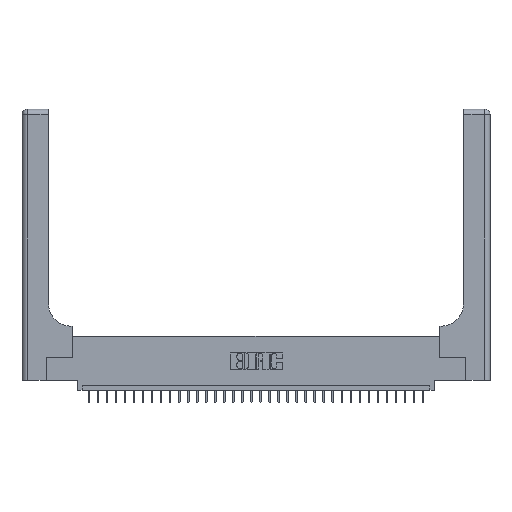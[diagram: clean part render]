
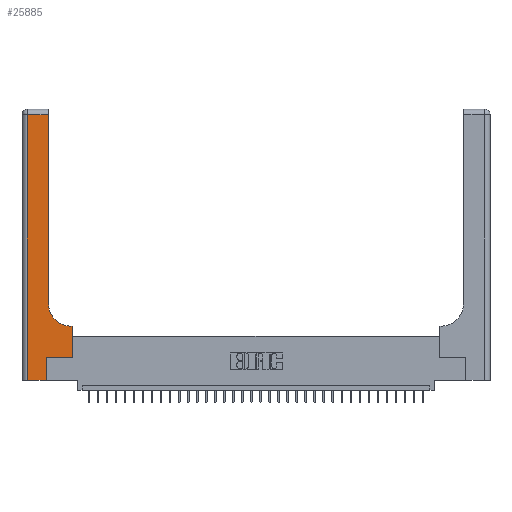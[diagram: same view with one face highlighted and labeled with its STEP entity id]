
A CAD part, top view. The second image highlights one B-rep face of the part: STEP entity #25885.
In plain terms, the highlighted planar face has unit normal (0, 0, 1).
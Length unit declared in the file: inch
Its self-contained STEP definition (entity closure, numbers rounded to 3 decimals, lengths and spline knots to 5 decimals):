
#152 = CARTESIAN_POINT ( 'NONE',  ( 0.2915, 0.6, 0.37 ) ) ;
#460 = EDGE_LOOP ( 'NONE', ( #8444, #33985, #28691, #29464, #1992, #9647, #3432, #23679, #12489 ) ) ;
#1067 = LINE ( 'NONE', #4034, #13639 ) ;
#1220 = EDGE_CURVE ( 'NONE', #16146, #11317, #33413, .T. ) ;
#1992 = ORIENTED_EDGE ( 'NONE', *, *, #14530, .T. ) ;
#2095 = CARTESIAN_POINT ( 'NONE',  ( 0.5585, 0.6, 0.37 ) ) ;
#3432 = ORIENTED_EDGE ( 'NONE', *, *, #22307, .T. ) ;
#3467 = DIRECTION ( 'NONE',  ( -1., 0., 0. ) ) ;
#3985 = EDGE_CURVE ( 'NONE', #18827, #16146, #16066, .T. ) ;
#3989 = VERTEX_POINT ( 'NONE', #16239 ) ;
#4034 = CARTESIAN_POINT ( 'NONE',  ( 0.2915, 3., 0.37 ) ) ;
#4475 = CARTESIAN_POINT ( 'NONE',  ( 0.5585, 0.25, 0.37 ) ) ;
#4802 = VERTEX_POINT ( 'NONE', #25611 ) ;
#5117 = CARTESIAN_POINT ( 'NONE',  ( 0.5415, 0.6, 0.37 ) ) ;
#5521 = VECTOR ( 'NONE', #21735, 39.37008 ) ;
#6195 = VECTOR ( 'NONE', #20926, 39.37008 ) ;
#6320 = LINE ( 'NONE', #27493, #5521 ) ;
#6955 = DIRECTION ( 'NONE',  ( -1., 0., 0. ) ) ;
#7333 = DIRECTION ( 'NONE',  ( 0., 0., -1. ) ) ;
#8444 = ORIENTED_EDGE ( 'NONE', *, *, #17525, .T. ) ;
#9647 = ORIENTED_EDGE ( 'NONE', *, *, #22580, .T. ) ;
#11091 = DIRECTION ( 'NONE',  ( 1., 0., 0. ) ) ;
#11154 = CARTESIAN_POINT ( 'NONE',  ( 0.06, 2.94, 0.37 ) ) ;
#11214 = EDGE_CURVE ( 'NONE', #3989, #29054, #6320, .T. ) ;
#11317 = VERTEX_POINT ( 'NONE', #25552 ) ;
#12489 = ORIENTED_EDGE ( 'NONE', *, *, #1220, .T. ) ;
#13508 = VERTEX_POINT ( 'NONE', #31583 ) ;
#13549 = EDGE_CURVE ( 'NONE', #13508, #22696, #31760, .T. ) ;
#13639 = VECTOR ( 'NONE', #27651, 39.37008 ) ;
#14232 = LINE ( 'NONE', #24223, #28880 ) ;
#14388 = CARTESIAN_POINT ( 'NONE',  ( 0.269, 0., 0.37 ) ) ;
#14448 = LINE ( 'NONE', #4475, #17110 ) ;
#14530 = EDGE_CURVE ( 'NONE', #22696, #4802, #32590, .T. ) ;
#14735 = CARTESIAN_POINT ( 'NONE',  ( 0.06, 3., 0.37 ) ) ;
#15183 = FACE_OUTER_BOUND ( 'NONE', #460, .T. ) ;
#15884 = EDGE_CURVE ( 'NONE', #29054, #13508, #17178, .T. ) ;
#16066 = LINE ( 'NONE', #152, #20074 ) ;
#16146 = VERTEX_POINT ( 'NONE', #5117 ) ;
#16239 = CARTESIAN_POINT ( 'NONE',  ( 0.2915, 2.94, 0.37 ) ) ;
#17110 = VECTOR ( 'NONE', #17749, 39.37008 ) ;
#17178 = LINE ( 'NONE', #14735, #30311 ) ;
#17525 = EDGE_CURVE ( 'NONE', #11317, #3989, #1067, .T. ) ;
#17749 = DIRECTION ( 'NONE',  ( 0., 1., 0. ) ) ;
#18466 = CARTESIAN_POINT ( 'NONE',  ( 0., 0., 0.37 ) ) ;
#18827 = VERTEX_POINT ( 'NONE', #2095 ) ;
#20074 = VECTOR ( 'NONE', #3467, 39.37008 ) ;
#20926 = DIRECTION ( 'NONE',  ( 1., 0., 0. ) ) ;
#21735 = DIRECTION ( 'NONE',  ( -1., 0., 0. ) ) ;
#21893 = VECTOR ( 'NONE', #22095, 39.37008 ) ;
#22095 = DIRECTION ( 'NONE',  ( 0., 1., 0. ) ) ;
#22205 = CARTESIAN_POINT ( 'NONE',  ( 0.5585, 0.25, 0.37 ) ) ;
#22307 = EDGE_CURVE ( 'NONE', #24770, #18827, #14448, .T. ) ;
#22580 = EDGE_CURVE ( 'NONE', #4802, #24770, #14232, .T. ) ;
#22696 = VERTEX_POINT ( 'NONE', #25415 ) ;
#22881 = PLANE ( 'NONE',  #33135 ) ;
#23679 = ORIENTED_EDGE ( 'NONE', *, *, #3985, .T. ) ;
#23955 = AXIS2_PLACEMENT_3D ( 'NONE', #31287, #7333, #28835 ) ;
#24223 = CARTESIAN_POINT ( 'NONE',  ( 0.269, 0.25, 0.37 ) ) ;
#24770 = VERTEX_POINT ( 'NONE', #22205 ) ;
#25415 = CARTESIAN_POINT ( 'NONE',  ( 0.269, 0., 0.37 ) ) ;
#25552 = CARTESIAN_POINT ( 'NONE',  ( 0.2915, 0.85, 0.37 ) ) ;
#25611 = CARTESIAN_POINT ( 'NONE',  ( 0.269, 0.25, 0.37 ) ) ;
#25885 = ADVANCED_FACE ( 'NONE', ( #15183 ), #22881, .F. ) ;
#27493 = CARTESIAN_POINT ( 'NONE',  ( 0., 2.94, 0.37 ) ) ;
#27651 = DIRECTION ( 'NONE',  ( 0., 1., 0. ) ) ;
#28691 = ORIENTED_EDGE ( 'NONE', *, *, #15884, .T. ) ;
#28835 = DIRECTION ( 'NONE',  ( 1., 0., 0. ) ) ;
#28880 = VECTOR ( 'NONE', #11091, 39.37008 ) ;
#29054 = VERTEX_POINT ( 'NONE', #11154 ) ;
#29464 = ORIENTED_EDGE ( 'NONE', *, *, #13549, .T. ) ;
#30133 = DIRECTION ( 'NONE',  ( 0., -1., 0. ) ) ;
#30311 = VECTOR ( 'NONE', #30133, 39.37008 ) ;
#30920 = DIRECTION ( 'NONE',  ( 0., 0., -1. ) ) ;
#31287 = CARTESIAN_POINT ( 'NONE',  ( 0.5415, 0.85, 0.37 ) ) ;
#31583 = CARTESIAN_POINT ( 'NONE',  ( 0.06, 0., 0.37 ) ) ;
#31760 = LINE ( 'NONE', #18466, #6195 ) ;
#32590 = LINE ( 'NONE', #14388, #21893 ) ;
#33135 = AXIS2_PLACEMENT_3D ( 'NONE', #33530, #30920, #6955 ) ;
#33413 = CIRCLE ( 'NONE', #23955, 0.25 ) ;
#33530 = CARTESIAN_POINT ( 'NONE',  ( 0., 3., 0.37 ) ) ;
#33985 = ORIENTED_EDGE ( 'NONE', *, *, #11214, .T. ) ;
